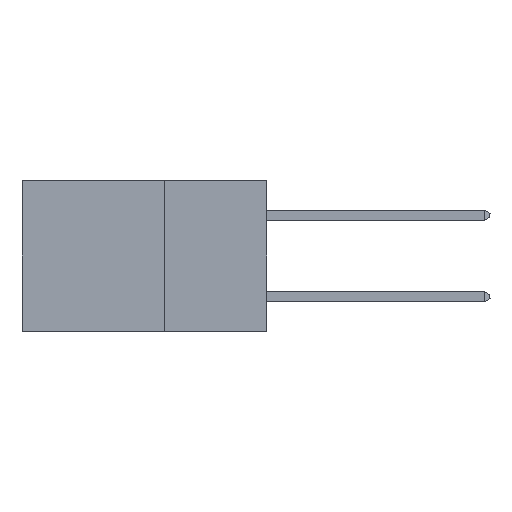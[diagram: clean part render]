
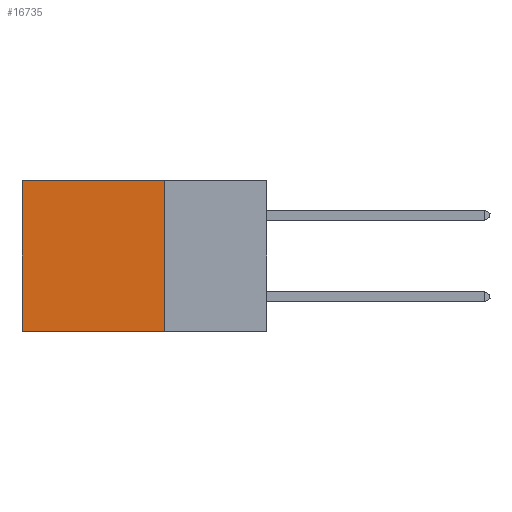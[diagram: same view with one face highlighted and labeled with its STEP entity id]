
A CAD part, left-side view. The second image highlights one B-rep face of the part: STEP entity #16735.
In plain terms, the highlighted planar face has unit normal (-1, 0, 0).
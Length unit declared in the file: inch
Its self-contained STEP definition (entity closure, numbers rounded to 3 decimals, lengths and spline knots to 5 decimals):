
#167 = DIRECTION ( 'NONE',  ( 0., 0., -1. ) ) ;
#498 = LINE ( 'NONE', #1324, #5661 ) ;
#1324 = CARTESIAN_POINT ( 'NONE',  ( 0.2875, 0.25, 0. ) ) ;
#1885 = ORIENTED_EDGE ( 'NONE', *, *, #17654, .F. ) ;
#1899 = VECTOR ( 'NONE', #7903, 39.37008 ) ;
#2052 = CARTESIAN_POINT ( 'NONE',  ( 0.2875, 0.25, 0. ) ) ;
#3596 = EDGE_CURVE ( 'NONE', #8006, #22425, #7046, .T. ) ;
#5661 = VECTOR ( 'NONE', #14749, 39.37008 ) ;
#6141 = CARTESIAN_POINT ( 'NONE',  ( 0.2875, 0.25, -0.37 ) ) ;
#6404 = EDGE_LOOP ( 'NONE', ( #6654, #16157, #1885, #11623 ) ) ;
#6654 = ORIENTED_EDGE ( 'NONE', *, *, #3596, .T. ) ;
#7046 = LINE ( 'NONE', #22812, #1899 ) ;
#7372 = EDGE_CURVE ( 'NONE', #15214, #8006, #15196, .T. ) ;
#7903 = DIRECTION ( 'NONE',  ( 0., 0., -1. ) ) ;
#8006 = VERTEX_POINT ( 'NONE', #16446 ) ;
#8565 = CARTESIAN_POINT ( 'NONE',  ( 0.2875, 0.25, -0.37 ) ) ;
#9555 = VECTOR ( 'NONE', #22034, 39.37008 ) ;
#10591 = DIRECTION ( 'NONE',  ( 0., 1., 0. ) ) ;
#11623 = ORIENTED_EDGE ( 'NONE', *, *, #7372, .T. ) ;
#11739 = DIRECTION ( 'NONE',  ( 1., 0., 0. ) ) ;
#12169 = LINE ( 'NONE', #8565, #16610 ) ;
#13065 = EDGE_CURVE ( 'NONE', #14028, #22425, #12169, .T. ) ;
#14028 = VERTEX_POINT ( 'NONE', #6141 ) ;
#14749 = DIRECTION ( 'NONE',  ( 0., 0., -1. ) ) ;
#15191 = CARTESIAN_POINT ( 'NONE',  ( 0.2875, 0.6, -0.37 ) ) ;
#15196 = LINE ( 'NONE', #18368, #9555 ) ;
#15214 = VERTEX_POINT ( 'NONE', #18973 ) ;
#16157 = ORIENTED_EDGE ( 'NONE', *, *, #13065, .F. ) ;
#16446 = CARTESIAN_POINT ( 'NONE',  ( 0.2875, 0.6, 0. ) ) ;
#16610 = VECTOR ( 'NONE', #10591, 39.37008 ) ;
#16735 = ADVANCED_FACE ( 'NONE', ( #17028 ), #17326, .F. ) ;
#17028 = FACE_OUTER_BOUND ( 'NONE', #6404, .T. ) ;
#17326 = PLANE ( 'NONE',  #20019 ) ;
#17654 = EDGE_CURVE ( 'NONE', #15214, #14028, #498, .T. ) ;
#18368 = CARTESIAN_POINT ( 'NONE',  ( 0.2875, 0.25, 0. ) ) ;
#18973 = CARTESIAN_POINT ( 'NONE',  ( 0.2875, 0.25, 0. ) ) ;
#20019 = AXIS2_PLACEMENT_3D ( 'NONE', #2052, #11739, #167 ) ;
#22034 = DIRECTION ( 'NONE',  ( 0., 1., 0. ) ) ;
#22425 = VERTEX_POINT ( 'NONE', #15191 ) ;
#22812 = CARTESIAN_POINT ( 'NONE',  ( 0.2875, 0.6, 0. ) ) ;
